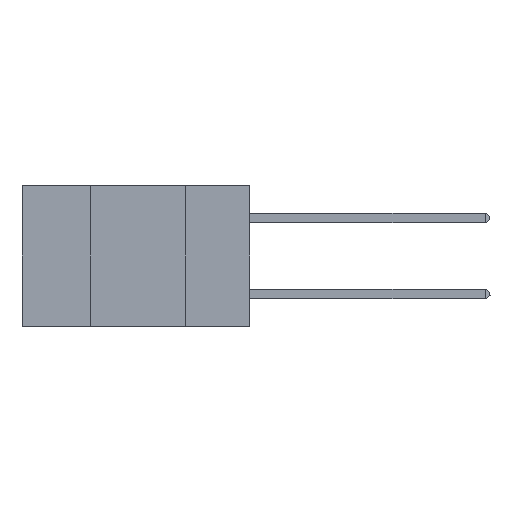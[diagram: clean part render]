
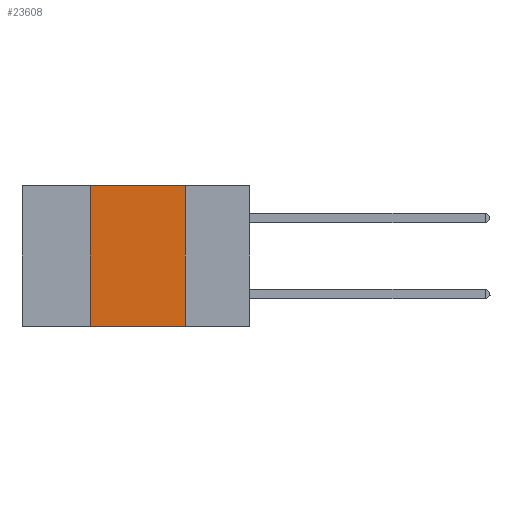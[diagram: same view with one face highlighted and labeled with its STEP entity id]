
A CAD part, left-side view. The second image highlights one B-rep face of the part: STEP entity #23608.
In plain terms, the highlighted planar face has unit normal (-1, 0, 0).
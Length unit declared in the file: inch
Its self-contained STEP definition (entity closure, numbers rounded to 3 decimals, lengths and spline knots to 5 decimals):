
#354 = EDGE_CURVE ( 'NONE', #13857, #14004, #20603, .T. ) ;
#1247 = CARTESIAN_POINT ( 'NONE',  ( 0., 0.17, 0. ) ) ;
#3474 = PLANE ( 'NONE',  #18400 ) ;
#3992 = CARTESIAN_POINT ( 'NONE',  ( 0., 0.17, -0.37 ) ) ;
#4801 = LINE ( 'NONE', #18692, #18271 ) ;
#6033 = FACE_OUTER_BOUND ( 'NONE', #24804, .T. ) ;
#6378 = ORIENTED_EDGE ( 'NONE', *, *, #8943, .F. ) ;
#7536 = VECTOR ( 'NONE', #9383, 39.37008 ) ;
#7574 = DIRECTION ( 'NONE',  ( 0., 0., -1. ) ) ;
#7748 = EDGE_CURVE ( 'NONE', #16471, #10916, #4801, .T. ) ;
#7756 = CARTESIAN_POINT ( 'NONE',  ( 0., 0.6, -0.37 ) ) ;
#8943 = EDGE_CURVE ( 'NONE', #10916, #14004, #19134, .T. ) ;
#9383 = DIRECTION ( 'NONE',  ( 0., 0., -1. ) ) ;
#9757 = CARTESIAN_POINT ( 'NONE',  ( 0., 0.6, 0. ) ) ;
#9900 = CARTESIAN_POINT ( 'NONE',  ( 0., 0.17, 0. ) ) ;
#10916 = VERTEX_POINT ( 'NONE', #9900 ) ;
#11408 = CARTESIAN_POINT ( 'NONE',  ( 0., 0.42, 0. ) ) ;
#11631 = DIRECTION ( 'NONE',  ( 1., 0., 0. ) ) ;
#12824 = ORIENTED_EDGE ( 'NONE', *, *, #7748, .F. ) ;
#13398 = VECTOR ( 'NONE', #13749, 39.37008 ) ;
#13749 = DIRECTION ( 'NONE',  ( 0., -1., 0. ) ) ;
#13857 = VERTEX_POINT ( 'NONE', #15818 ) ;
#14004 = VERTEX_POINT ( 'NONE', #3992 ) ;
#15818 = CARTESIAN_POINT ( 'NONE',  ( 0., 0.42, -0.37 ) ) ;
#15846 = LINE ( 'NONE', #11408, #21795 ) ;
#16471 = VERTEX_POINT ( 'NONE', #18612 ) ;
#18271 = VECTOR ( 'NONE', #22618, 39.37008 ) ;
#18400 = AXIS2_PLACEMENT_3D ( 'NONE', #9757, #11631, #7574 ) ;
#18612 = CARTESIAN_POINT ( 'NONE',  ( 0., 0.42, 0. ) ) ;
#18692 = CARTESIAN_POINT ( 'NONE',  ( 0., 0.6, 0. ) ) ;
#19134 = LINE ( 'NONE', #1247, #7536 ) ;
#20603 = LINE ( 'NONE', #7756, #13398 ) ;
#21795 = VECTOR ( 'NONE', #25431, 39.37008 ) ;
#21946 = EDGE_CURVE ( 'NONE', #13857, #16471, #15846, .T. ) ;
#22618 = DIRECTION ( 'NONE',  ( 0., -1., 0. ) ) ;
#23608 = ADVANCED_FACE ( 'NONE', ( #6033 ), #3474, .F. ) ;
#24764 = ORIENTED_EDGE ( 'NONE', *, *, #354, .T. ) ;
#24804 = EDGE_LOOP ( 'NONE', ( #6378, #12824, #25129, #24764 ) ) ;
#25129 = ORIENTED_EDGE ( 'NONE', *, *, #21946, .F. ) ;
#25431 = DIRECTION ( 'NONE',  ( 0., 0., 1. ) ) ;
